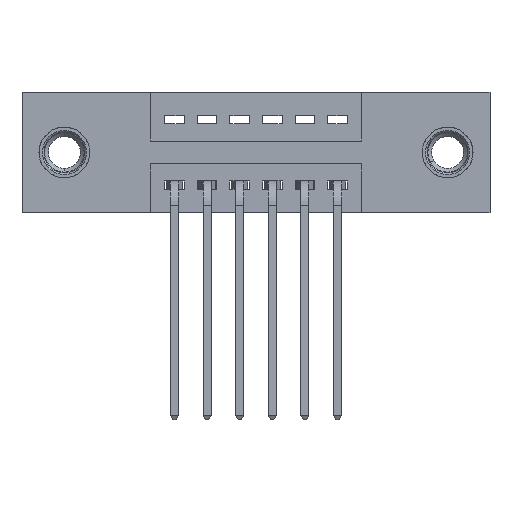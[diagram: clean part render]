
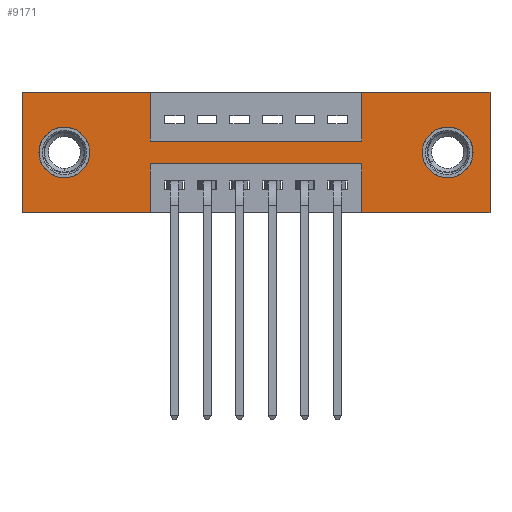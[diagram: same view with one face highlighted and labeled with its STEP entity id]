
A CAD part, front view. The second image highlights one B-rep face of the part: STEP entity #9171.
In plain terms, the highlighted planar face has unit normal (0, -1, 0).
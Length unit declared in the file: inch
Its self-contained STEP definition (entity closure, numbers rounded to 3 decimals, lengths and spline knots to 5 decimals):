
#359 = CARTESIAN_POINT ( 'NONE',  ( 0., 0., -0.37 ) ) ;
#391 = EDGE_CURVE ( 'NONE', #5037, #3291, #3329, .T. ) ;
#520 = LINE ( 'NONE', #2410, #7202 ) ;
#530 = CARTESIAN_POINT ( 'NONE',  ( 1.435, 0., 0. ) ) ;
#599 = DIRECTION ( 'NONE',  ( 0., 0., -1. ) ) ;
#642 = AXIS2_PLACEMENT_3D ( 'NONE', #1316, #7181, #10362 ) ;
#837 = CARTESIAN_POINT ( 'NONE',  ( 1.0425, 0., 0. ) ) ;
#993 = LINE ( 'NONE', #7380, #2138 ) ;
#1005 = VECTOR ( 'NONE', #4231, 39.37008 ) ;
#1316 = CARTESIAN_POINT ( 'NONE',  ( 0.13, 0., -0.185 ) ) ;
#1501 = DIRECTION ( 'NONE',  ( 0., 0., -1. ) ) ;
#1581 = DIRECTION ( 'NONE',  ( 1., 0., 0. ) ) ;
#1601 = VECTOR ( 'NONE', #6296, 39.37008 ) ;
#1620 = EDGE_CURVE ( 'NONE', #2479, #5037, #3689, .T. ) ;
#1651 = DIRECTION ( 'NONE',  ( 0., 0., -1. ) ) ;
#1794 = CARTESIAN_POINT ( 'NONE',  ( 0.3925, 0., -0.22 ) ) ;
#1802 = CARTESIAN_POINT ( 'NONE',  ( 0., 0., -0.37 ) ) ;
#1852 = ORIENTED_EDGE ( 'NONE', *, *, #5767, .F. ) ;
#1877 = CARTESIAN_POINT ( 'NONE',  ( 0., 0., -0.37 ) ) ;
#1906 = DIRECTION ( 'NONE',  ( 0., 0., -1. ) ) ;
#2028 = EDGE_CURVE ( 'NONE', #8088, #10626, #3338, .T. ) ;
#2127 = VECTOR ( 'NONE', #7699, 39.37008 ) ;
#2138 = VECTOR ( 'NONE', #1651, 39.37008 ) ;
#2410 = CARTESIAN_POINT ( 'NONE',  ( 1.0425, 0., -0.37 ) ) ;
#2479 = VERTEX_POINT ( 'NONE', #5461 ) ;
#2527 = CARTESIAN_POINT ( 'NONE',  ( 0., 0., 0. ) ) ;
#2571 = ORIENTED_EDGE ( 'NONE', *, *, #7006, .F. ) ;
#2605 = VERTEX_POINT ( 'NONE', #3229 ) ;
#2636 = AXIS2_PLACEMENT_3D ( 'NONE', #10510, #5622, #599 ) ;
#2723 = CARTESIAN_POINT ( 'NONE',  ( 0.3925, 0., -0.22 ) ) ;
#2827 = VECTOR ( 'NONE', #1581, 39.37008 ) ;
#2857 = ORIENTED_EDGE ( 'NONE', *, *, #1620, .F. ) ;
#2918 = ORIENTED_EDGE ( 'NONE', *, *, #9307, .F. ) ;
#3128 = VECTOR ( 'NONE', #7241, 39.37008 ) ;
#3229 = CARTESIAN_POINT ( 'NONE',  ( 1.0425, 0., -0.37 ) ) ;
#3291 = VERTEX_POINT ( 'NONE', #5382 ) ;
#3329 = LINE ( 'NONE', #2527, #1005 ) ;
#3338 = LINE ( 'NONE', #6544, #2827 ) ;
#3376 = VERTEX_POINT ( 'NONE', #7936 ) ;
#3377 = CARTESIAN_POINT ( 'NONE',  ( 0.3925, 0., 0. ) ) ;
#3446 = EDGE_CURVE ( 'NONE', #7340, #6895, #8497, .T. ) ;
#3523 = VERTEX_POINT ( 'NONE', #5620 ) ;
#3547 = CIRCLE ( 'NONE', #642, 0.078 ) ;
#3548 = VECTOR ( 'NONE', #5249, 39.37008 ) ;
#3634 = EDGE_LOOP ( 'NONE', ( #7690, #7067 ) ) ;
#3646 = VERTEX_POINT ( 'NONE', #2723 ) ;
#3650 = CARTESIAN_POINT ( 'NONE',  ( 0.13, 0., -0.185 ) ) ;
#3667 = CIRCLE ( 'NONE', #2636, 0.078 ) ;
#3689 = LINE ( 'NONE', #1802, #4977 ) ;
#3762 = ORIENTED_EDGE ( 'NONE', *, *, #8485, .F. ) ;
#3792 = LINE ( 'NONE', #530, #1601 ) ;
#3814 = AXIS2_PLACEMENT_3D ( 'NONE', #10233, #4542, #1906 ) ;
#3828 = EDGE_CURVE ( 'NONE', #2605, #3523, #520, .T. ) ;
#4076 = ORIENTED_EDGE ( 'NONE', *, *, #5010, .F. ) ;
#4112 = VECTOR ( 'NONE', #10092, 39.37008 ) ;
#4231 = DIRECTION ( 'NONE',  ( 0., 0., 1. ) ) ;
#4489 = VERTEX_POINT ( 'NONE', #7737 ) ;
#4542 = DIRECTION ( 'NONE',  ( 0., -1., 0. ) ) ;
#4641 = VERTEX_POINT ( 'NONE', #8833 ) ;
#4661 = CARTESIAN_POINT ( 'NONE',  ( 1.0425, 0., -0.15 ) ) ;
#4876 = CARTESIAN_POINT ( 'NONE',  ( 1.305, 0., -0.107 ) ) ;
#4977 = VECTOR ( 'NONE', #5928, 39.37008 ) ;
#4997 = ORIENTED_EDGE ( 'NONE', *, *, #391, .F. ) ;
#5010 = EDGE_CURVE ( 'NONE', #3523, #3646, #8970, .T. ) ;
#5037 = VERTEX_POINT ( 'NONE', #359 ) ;
#5249 = DIRECTION ( 'NONE',  ( -1., 0., 0. ) ) ;
#5382 = CARTESIAN_POINT ( 'NONE',  ( 0., 0., 0. ) ) ;
#5383 = VECTOR ( 'NONE', #9429, 39.37008 ) ;
#5461 = CARTESIAN_POINT ( 'NONE',  ( 0.3925, 0., -0.37 ) ) ;
#5505 = FACE_BOUND ( 'NONE', #3634, .T. ) ;
#5532 = AXIS2_PLACEMENT_3D ( 'NONE', #7971, #10470, #1501 ) ;
#5620 = CARTESIAN_POINT ( 'NONE',  ( 1.0425, 0., -0.22 ) ) ;
#5622 = DIRECTION ( 'NONE',  ( 0., 1., 0. ) ) ;
#5767 = EDGE_CURVE ( 'NONE', #3646, #2479, #993, .T. ) ;
#5928 = DIRECTION ( 'NONE',  ( -1., 0., 0. ) ) ;
#5966 = ORIENTED_EDGE ( 'NONE', *, *, #6377, .T. ) ;
#6068 = VERTEX_POINT ( 'NONE', #837 ) ;
#6235 = CARTESIAN_POINT ( 'NONE',  ( 0.3925, 0., -0.15 ) ) ;
#6296 = DIRECTION ( 'NONE',  ( 0., 0., -1. ) ) ;
#6324 = EDGE_CURVE ( 'NONE', #6068, #3376, #9202, .T. ) ;
#6377 = EDGE_CURVE ( 'NONE', #4489, #4641, #8317, .T. ) ;
#6544 = CARTESIAN_POINT ( 'NONE',  ( 0.3925, 0., -0.15 ) ) ;
#6616 = AXIS2_PLACEMENT_3D ( 'NONE', #3650, #10306, #9390 ) ;
#6733 = EDGE_CURVE ( 'NONE', #8323, #2605, #8172, .T. ) ;
#6783 = ORIENTED_EDGE ( 'NONE', *, *, #2028, .F. ) ;
#6895 = VERTEX_POINT ( 'NONE', #10304 ) ;
#6915 = PLANE ( 'NONE',  #3814 ) ;
#6980 = CARTESIAN_POINT ( 'NONE',  ( 0., 0., 0. ) ) ;
#7006 = EDGE_CURVE ( 'NONE', #3376, #8323, #3792, .T. ) ;
#7024 = EDGE_LOOP ( 'NONE', ( #5966, #7867 ) ) ;
#7067 = ORIENTED_EDGE ( 'NONE', *, *, #7235, .T. ) ;
#7181 = DIRECTION ( 'NONE',  ( 0., 1., 0. ) ) ;
#7202 = VECTOR ( 'NONE', #8915, 39.37008 ) ;
#7235 = EDGE_CURVE ( 'NONE', #6895, #7340, #3667, .T. ) ;
#7241 = DIRECTION ( 'NONE',  ( 0., 0., 1. ) ) ;
#7288 = FACE_OUTER_BOUND ( 'NONE', #8958, .T. ) ;
#7340 = VERTEX_POINT ( 'NONE', #4876 ) ;
#7341 = CARTESIAN_POINT ( 'NONE',  ( 1.435, 0., -0.37 ) ) ;
#7380 = CARTESIAN_POINT ( 'NONE',  ( 0.3925, 0., -0.37 ) ) ;
#7690 = ORIENTED_EDGE ( 'NONE', *, *, #3446, .T. ) ;
#7699 = DIRECTION ( 'NONE',  ( 1., 0., 0. ) ) ;
#7737 = CARTESIAN_POINT ( 'NONE',  ( 0.13, 0., -0.107 ) ) ;
#7744 = ORIENTED_EDGE ( 'NONE', *, *, #9132, .F. ) ;
#7786 = VECTOR ( 'NONE', #8771, 39.37008 ) ;
#7867 = ORIENTED_EDGE ( 'NONE', *, *, #9924, .T. ) ;
#7936 = CARTESIAN_POINT ( 'NONE',  ( 1.435, 0., 0. ) ) ;
#7971 = CARTESIAN_POINT ( 'NONE',  ( 1.305, 0., -0.185 ) ) ;
#8088 = VERTEX_POINT ( 'NONE', #6235 ) ;
#8172 = LINE ( 'NONE', #1877, #3548 ) ;
#8317 = CIRCLE ( 'NONE', #6616, 0.078 ) ;
#8323 = VERTEX_POINT ( 'NONE', #7341 ) ;
#8485 = EDGE_CURVE ( 'NONE', #10626, #6068, #9935, .T. ) ;
#8497 = CIRCLE ( 'NONE', #5532, 0.078 ) ;
#8737 = CARTESIAN_POINT ( 'NONE',  ( 0., 0., 0. ) ) ;
#8769 = ORIENTED_EDGE ( 'NONE', *, *, #3828, .F. ) ;
#8771 = DIRECTION ( 'NONE',  ( 1., 0., 0. ) ) ;
#8833 = CARTESIAN_POINT ( 'NONE',  ( 0.13, 0., -0.263 ) ) ;
#8915 = DIRECTION ( 'NONE',  ( 0., 0., 1. ) ) ;
#8958 = EDGE_LOOP ( 'NONE', ( #1852, #4076, #8769, #9814, #2571, #9521, #3762, #6783, #7744, #2918, #4997, #2857 ) ) ;
#8970 = LINE ( 'NONE', #1794, #4112 ) ;
#9132 = EDGE_CURVE ( 'NONE', #9612, #8088, #10605, .T. ) ;
#9171 = ADVANCED_FACE ( 'NONE', ( #5505, #9850, #7288 ), #6915, .T. ) ;
#9202 = LINE ( 'NONE', #6980, #2127 ) ;
#9307 = EDGE_CURVE ( 'NONE', #3291, #9612, #9968, .T. ) ;
#9390 = DIRECTION ( 'NONE',  ( 0., 0., 1. ) ) ;
#9407 = CARTESIAN_POINT ( 'NONE',  ( 1.0425, 0., 0. ) ) ;
#9429 = DIRECTION ( 'NONE',  ( 0., 0., -1. ) ) ;
#9521 = ORIENTED_EDGE ( 'NONE', *, *, #6324, .F. ) ;
#9612 = VERTEX_POINT ( 'NONE', #3377 ) ;
#9814 = ORIENTED_EDGE ( 'NONE', *, *, #6733, .F. ) ;
#9850 = FACE_BOUND ( 'NONE', #7024, .T. ) ;
#9924 = EDGE_CURVE ( 'NONE', #4641, #4489, #3547, .T. ) ;
#9935 = LINE ( 'NONE', #9407, #3128 ) ;
#9968 = LINE ( 'NONE', #8737, #7786 ) ;
#10092 = DIRECTION ( 'NONE',  ( -1., 0., 0. ) ) ;
#10203 = CARTESIAN_POINT ( 'NONE',  ( 0.3925, 0., 0. ) ) ;
#10233 = CARTESIAN_POINT ( 'NONE',  ( 0., 0., -0.37 ) ) ;
#10304 = CARTESIAN_POINT ( 'NONE',  ( 1.305, 0., -0.263 ) ) ;
#10306 = DIRECTION ( 'NONE',  ( 0., 1., 0. ) ) ;
#10362 = DIRECTION ( 'NONE',  ( 0., 0., 1. ) ) ;
#10470 = DIRECTION ( 'NONE',  ( 0., 1., 0. ) ) ;
#10510 = CARTESIAN_POINT ( 'NONE',  ( 1.305, 0., -0.185 ) ) ;
#10605 = LINE ( 'NONE', #10203, #5383 ) ;
#10626 = VERTEX_POINT ( 'NONE', #4661 ) ;
